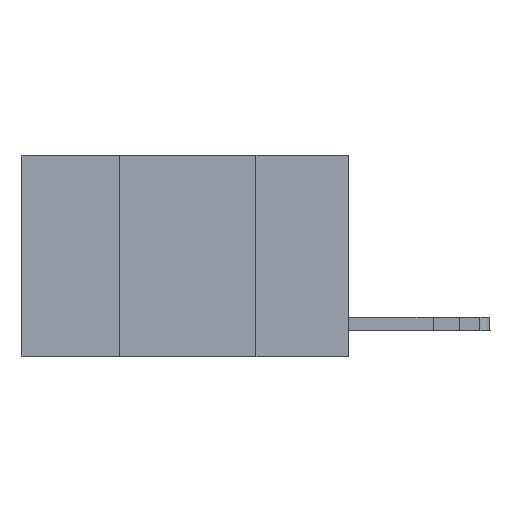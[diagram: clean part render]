
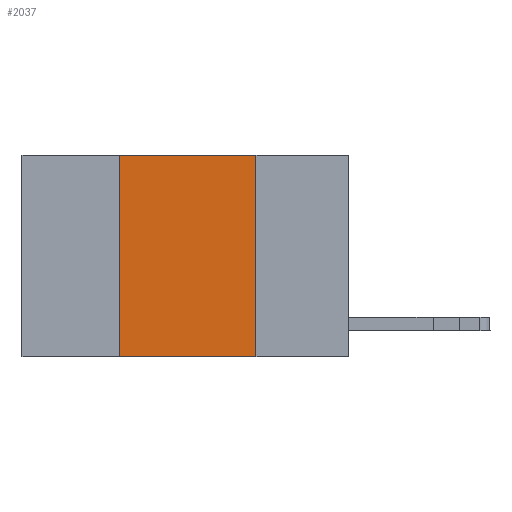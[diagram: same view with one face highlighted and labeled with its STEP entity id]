
A CAD part, left-side view. The second image highlights one B-rep face of the part: STEP entity #2037.
In plain terms, the highlighted planar face has unit normal (-1, 0, 0).
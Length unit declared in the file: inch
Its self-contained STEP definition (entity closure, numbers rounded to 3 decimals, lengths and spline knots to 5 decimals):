
#990 = VECTOR ( 'NONE', #7638, 39.37008 ) ;
#1406 = VERTEX_POINT ( 'NONE', #2004 ) ;
#2004 = CARTESIAN_POINT ( 'NONE',  ( 0., 0.17, 0. ) ) ;
#2037 = ADVANCED_FACE ( 'NONE', ( #9605 ), #6479, .F. ) ;
#4302 = CARTESIAN_POINT ( 'NONE',  ( 0., 0.42, -0.37 ) ) ;
#4306 = CARTESIAN_POINT ( 'NONE',  ( 0., 0.42, 0. ) ) ;
#4634 = DIRECTION ( 'NONE',  ( 0., 0., -1. ) ) ;
#5490 = EDGE_CURVE ( 'NONE', #11434, #1406, #10843, .T. ) ;
#5818 = CARTESIAN_POINT ( 'NONE',  ( 0., 0.6, -0.37 ) ) ;
#6036 = AXIS2_PLACEMENT_3D ( 'NONE', #9761, #10848, #4634 ) ;
#6479 = PLANE ( 'NONE',  #6036 ) ;
#6837 = DIRECTION ( 'NONE',  ( 0., -1., 0. ) ) ;
#7545 = VERTEX_POINT ( 'NONE', #4302 ) ;
#7638 = DIRECTION ( 'NONE',  ( 0., 0., -1. ) ) ;
#7669 = CARTESIAN_POINT ( 'NONE',  ( 0., 0.42, 0. ) ) ;
#8391 = ORIENTED_EDGE ( 'NONE', *, *, #5490, .F. ) ;
#8458 = EDGE_CURVE ( 'NONE', #1406, #10226, #11700, .T. ) ;
#8494 = EDGE_CURVE ( 'NONE', #7545, #11434, #11417, .T. ) ;
#8609 = EDGE_CURVE ( 'NONE', #7545, #10226, #12466, .T. ) ;
#8853 = ORIENTED_EDGE ( 'NONE', *, *, #8494, .F. ) ;
#8866 = VECTOR ( 'NONE', #12531, 39.37008 ) ;
#9605 = FACE_OUTER_BOUND ( 'NONE', #10527, .T. ) ;
#9761 = CARTESIAN_POINT ( 'NONE',  ( 0., 0.6, 0. ) ) ;
#10226 = VERTEX_POINT ( 'NONE', #10725 ) ;
#10320 = ORIENTED_EDGE ( 'NONE', *, *, #8458, .F. ) ;
#10527 = EDGE_LOOP ( 'NONE', ( #10320, #8391, #8853, #11520 ) ) ;
#10567 = VECTOR ( 'NONE', #12249, 39.37008 ) ;
#10725 = CARTESIAN_POINT ( 'NONE',  ( 0., 0.17, -0.37 ) ) ;
#10843 = LINE ( 'NONE', #12775, #10567 ) ;
#10848 = DIRECTION ( 'NONE',  ( 1., 0., 0. ) ) ;
#11417 = LINE ( 'NONE', #7669, #8866 ) ;
#11434 = VERTEX_POINT ( 'NONE', #4306 ) ;
#11518 = CARTESIAN_POINT ( 'NONE',  ( 0., 0.17, 0. ) ) ;
#11520 = ORIENTED_EDGE ( 'NONE', *, *, #8609, .T. ) ;
#11700 = LINE ( 'NONE', #11518, #990 ) ;
#12148 = VECTOR ( 'NONE', #6837, 39.37008 ) ;
#12249 = DIRECTION ( 'NONE',  ( 0., -1., 0. ) ) ;
#12466 = LINE ( 'NONE', #5818, #12148 ) ;
#12531 = DIRECTION ( 'NONE',  ( 0., 0., 1. ) ) ;
#12775 = CARTESIAN_POINT ( 'NONE',  ( 0., 0.6, 0. ) ) ;
